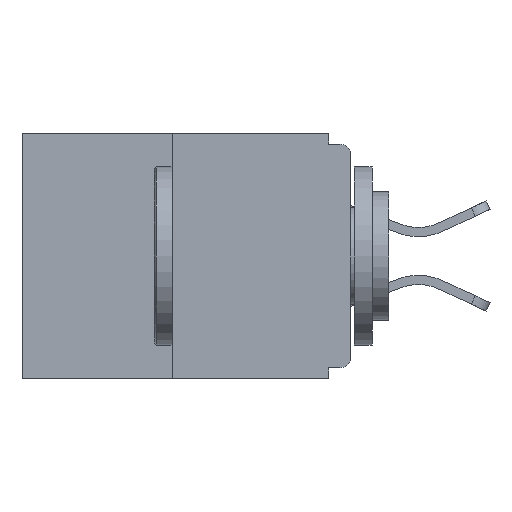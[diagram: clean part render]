
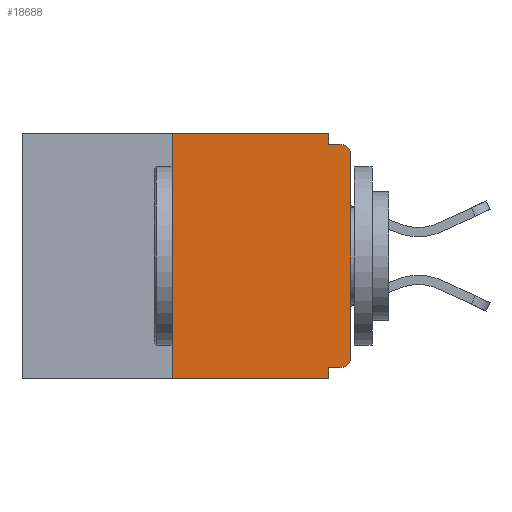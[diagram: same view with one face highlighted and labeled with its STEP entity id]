
A CAD part, left-side view. The second image highlights one B-rep face of the part: STEP entity #18688.
In plain terms, the highlighted planar face has unit normal (-1, 0, 0).
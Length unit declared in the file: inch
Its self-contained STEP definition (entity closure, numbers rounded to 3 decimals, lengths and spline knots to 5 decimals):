
#35 = AXIS2_PLACEMENT_3D ( 'NONE', #20177, #137, #16701 ) ;
#83 = VECTOR ( 'NONE', #17231, 39.37008 ) ;
#137 = DIRECTION ( 'NONE',  ( -1., 0., 0. ) ) ;
#634 = CARTESIAN_POINT ( 'NONE',  ( 0., 0.015, -0.015 ) ) ;
#939 = DIRECTION ( 'NONE',  ( 0., 0., -1. ) ) ;
#1105 = EDGE_LOOP ( 'NONE', ( #12553, #2055, #7565, #8053, #10751, #13548, #11964, #20906, #19305, #2053 ) ) ;
#1226 = CARTESIAN_POINT ( 'NONE',  ( 0., 0.46, 0. ) ) ;
#1392 = LINE ( 'NONE', #21117, #15585 ) ;
#1531 = DIRECTION ( 'NONE',  ( 1., 0., 0. ) ) ;
#1646 = EDGE_CURVE ( 'NONE', #7878, #12924, #5716, .T. ) ;
#2053 = ORIENTED_EDGE ( 'NONE', *, *, #12391, .F. ) ;
#2055 = ORIENTED_EDGE ( 'NONE', *, *, #15524, .F. ) ;
#2074 = CARTESIAN_POINT ( 'NONE',  ( 0., 0., -0.015 ) ) ;
#4167 = CARTESIAN_POINT ( 'NONE',  ( 0., 0.031, -0.343 ) ) ;
#4286 = EDGE_CURVE ( 'NONE', #17269, #12676, #18552, .T. ) ;
#4726 = DIRECTION ( 'NONE',  ( 0., 0., 1. ) ) ;
#4851 = CARTESIAN_POINT ( 'NONE',  ( 0., 0.25, 0. ) ) ;
#5009 = CARTESIAN_POINT ( 'NONE',  ( 0., 0.031, -0.015 ) ) ;
#5017 = VECTOR ( 'NONE', #5517, 39.37008 ) ;
#5099 = DIRECTION ( 'NONE',  ( -1., 0., 0. ) ) ;
#5318 = EDGE_CURVE ( 'NONE', #12924, #12498, #1392, .T. ) ;
#5517 = DIRECTION ( 'NONE',  ( 0., -1., 0. ) ) ;
#5557 = CARTESIAN_POINT ( 'NONE',  ( 0., 0., -0.328 ) ) ;
#5605 = EDGE_CURVE ( 'NONE', #14300, #7523, #9233, .T. ) ;
#5716 = CIRCLE ( 'NONE', #15866, 0.015 ) ;
#6267 = CARTESIAN_POINT ( 'NONE',  ( 0., 0., -0.313 ) ) ;
#6344 = LINE ( 'NONE', #15534, #83 ) ;
#6465 = EDGE_CURVE ( 'NONE', #12498, #15684, #11586, .T. ) ;
#6501 = CARTESIAN_POINT ( 'NONE',  ( 0., 0.46, 0. ) ) ;
#6873 = CARTESIAN_POINT ( 'NONE',  ( 0., 0.031, 0. ) ) ;
#6890 = LINE ( 'NONE', #5557, #11698 ) ;
#7116 = FACE_OUTER_BOUND ( 'NONE', #1105, .T. ) ;
#7250 = EDGE_CURVE ( 'NONE', #14871, #15684, #18965, .T. ) ;
#7523 = VERTEX_POINT ( 'NONE', #21666 ) ;
#7565 = ORIENTED_EDGE ( 'NONE', *, *, #13889, .T. ) ;
#7635 = DIRECTION ( 'NONE',  ( 0., 1., 0. ) ) ;
#7878 = VERTEX_POINT ( 'NONE', #14430 ) ;
#8010 = VECTOR ( 'NONE', #8129, 39.37008 ) ;
#8053 = ORIENTED_EDGE ( 'NONE', *, *, #5605, .F. ) ;
#8129 = DIRECTION ( 'NONE',  ( 0., -1., 0. ) ) ;
#9233 = LINE ( 'NONE', #4167, #18993 ) ;
#9522 = DIRECTION ( 'NONE',  ( 0., 0., 1. ) ) ;
#9824 = VECTOR ( 'NONE', #11565, 39.37008 ) ;
#10751 = ORIENTED_EDGE ( 'NONE', *, *, #20977, .F. ) ;
#11241 = CARTESIAN_POINT ( 'NONE',  ( 0., 0., -0.03 ) ) ;
#11565 = DIRECTION ( 'NONE',  ( 0., 0., -1. ) ) ;
#11586 = CIRCLE ( 'NONE', #35, 0.015 ) ;
#11698 = VECTOR ( 'NONE', #7635, 39.37008 ) ;
#11955 = LINE ( 'NONE', #15349, #9824 ) ;
#11964 = ORIENTED_EDGE ( 'NONE', *, *, #5318, .T. ) ;
#12391 = EDGE_CURVE ( 'NONE', #12676, #14871, #11955, .T. ) ;
#12498 = VERTEX_POINT ( 'NONE', #11241 ) ;
#12553 = ORIENTED_EDGE ( 'NONE', *, *, #4286, .F. ) ;
#12676 = VERTEX_POINT ( 'NONE', #6873 ) ;
#12924 = VERTEX_POINT ( 'NONE', #6267 ) ;
#13548 = ORIENTED_EDGE ( 'NONE', *, *, #1646, .T. ) ;
#13574 = VECTOR ( 'NONE', #4726, 39.37008 ) ;
#13889 = EDGE_CURVE ( 'NONE', #15449, #7523, #6344, .T. ) ;
#14300 = VERTEX_POINT ( 'NONE', #20434 ) ;
#14430 = CARTESIAN_POINT ( 'NONE',  ( 0., 0.015, -0.328 ) ) ;
#14556 = AXIS2_PLACEMENT_3D ( 'NONE', #1226, #1531, #18198 ) ;
#14814 = PLANE ( 'NONE',  #14556 ) ;
#14871 = VERTEX_POINT ( 'NONE', #5009 ) ;
#15166 = CARTESIAN_POINT ( 'NONE',  ( 0., 0.015, -0.313 ) ) ;
#15349 = CARTESIAN_POINT ( 'NONE',  ( 0., 0.031, 0. ) ) ;
#15449 = VERTEX_POINT ( 'NONE', #16320 ) ;
#15524 = EDGE_CURVE ( 'NONE', #15449, #17269, #17764, .T. ) ;
#15534 = CARTESIAN_POINT ( 'NONE',  ( 0., 0.46, -0.343 ) ) ;
#15585 = VECTOR ( 'NONE', #9522, 39.37008 ) ;
#15684 = VERTEX_POINT ( 'NONE', #634 ) ;
#15866 = AXIS2_PLACEMENT_3D ( 'NONE', #15166, #5099, #16844 ) ;
#16320 = CARTESIAN_POINT ( 'NONE',  ( 0., 0.25, -0.343 ) ) ;
#16701 = DIRECTION ( 'NONE',  ( 0., 0., -1. ) ) ;
#16844 = DIRECTION ( 'NONE',  ( 0., 0., -1. ) ) ;
#17231 = DIRECTION ( 'NONE',  ( 0., -1., 0. ) ) ;
#17269 = VERTEX_POINT ( 'NONE', #4851 ) ;
#17764 = LINE ( 'NONE', #18182, #13574 ) ;
#18182 = CARTESIAN_POINT ( 'NONE',  ( 0., 0.25, 0. ) ) ;
#18198 = DIRECTION ( 'NONE',  ( 0., 0., -1. ) ) ;
#18552 = LINE ( 'NONE', #6501, #8010 ) ;
#18688 = ADVANCED_FACE ( 'NONE', ( #7116 ), #14814, .F. ) ;
#18965 = LINE ( 'NONE', #2074, #5017 ) ;
#18993 = VECTOR ( 'NONE', #939, 39.37008 ) ;
#19305 = ORIENTED_EDGE ( 'NONE', *, *, #7250, .F. ) ;
#20177 = CARTESIAN_POINT ( 'NONE',  ( 0., 0.015, -0.03 ) ) ;
#20434 = CARTESIAN_POINT ( 'NONE',  ( 0., 0.031, -0.328 ) ) ;
#20906 = ORIENTED_EDGE ( 'NONE', *, *, #6465, .T. ) ;
#20977 = EDGE_CURVE ( 'NONE', #7878, #14300, #6890, .T. ) ;
#21117 = CARTESIAN_POINT ( 'NONE',  ( 0., 0., 0. ) ) ;
#21666 = CARTESIAN_POINT ( 'NONE',  ( 0., 0.031, -0.343 ) ) ;
